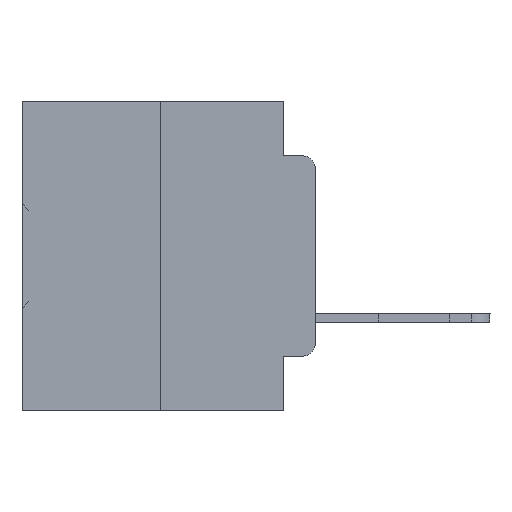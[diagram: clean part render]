
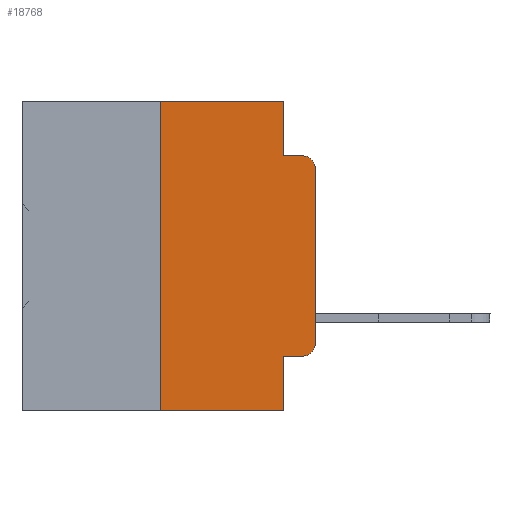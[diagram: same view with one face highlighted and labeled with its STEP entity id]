
A CAD part, left-side view. The second image highlights one B-rep face of the part: STEP entity #18768.
In plain terms, the highlighted planar face has unit normal (-1, 0, 0).
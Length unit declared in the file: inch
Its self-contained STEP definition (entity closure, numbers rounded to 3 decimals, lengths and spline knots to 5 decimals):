
#83 = EDGE_CURVE ( 'NONE', #33465, #11536, #35253, .T. ) ;
#577 = AXIS2_PLACEMENT_3D ( 'NONE', #12621, #35290, #26552 ) ;
#908 = CARTESIAN_POINT ( 'NONE',  ( 0., 0.473, 0. ) ) ;
#1136 = VERTEX_POINT ( 'NONE', #9105 ) ;
#1549 = LINE ( 'NONE', #27150, #31148 ) ;
#1655 = DIRECTION ( 'NONE',  ( 0., 0., -1. ) ) ;
#2420 = LINE ( 'NONE', #14021, #12284 ) ;
#2438 = ORIENTED_EDGE ( 'NONE', *, *, #31222, .T. ) ;
#2565 = DIRECTION ( 'NONE',  ( 0., 0., 1. ) ) ;
#2573 = LINE ( 'NONE', #4556, #23668 ) ;
#2904 = LINE ( 'NONE', #30087, #32514 ) ;
#3123 = AXIS2_PLACEMENT_3D ( 'NONE', #12083, #23395, #11851 ) ;
#3147 = VERTEX_POINT ( 'NONE', #8550 ) ;
#3445 = ORIENTED_EDGE ( 'NONE', *, *, #31385, .T. ) ;
#3495 = VERTEX_POINT ( 'NONE', #3893 ) ;
#3783 = DIRECTION ( 'NONE',  ( 1., 0., 0. ) ) ;
#3893 = CARTESIAN_POINT ( 'NONE',  ( 0., 0., -0.3915 ) ) ;
#4528 = ORIENTED_EDGE ( 'NONE', *, *, #83, .F. ) ;
#4556 = CARTESIAN_POINT ( 'NONE',  ( 0., 0.051, -0.0885 ) ) ;
#5218 = VECTOR ( 'NONE', #34963, 39.37008 ) ;
#6256 = VERTEX_POINT ( 'NONE', #10395 ) ;
#6557 = EDGE_CURVE ( 'NONE', #8669, #3147, #7519, .T. ) ;
#6685 = CARTESIAN_POINT ( 'NONE',  ( 0., 0.051, 0. ) ) ;
#7519 = LINE ( 'NONE', #17451, #8849 ) ;
#8210 = ORIENTED_EDGE ( 'NONE', *, *, #6557, .F. ) ;
#8270 = CARTESIAN_POINT ( 'NONE',  ( 0., 0.051, -0.0885 ) ) ;
#8550 = CARTESIAN_POINT ( 'NONE',  ( 0., 0.051, 0. ) ) ;
#8669 = VERTEX_POINT ( 'NONE', #10685 ) ;
#8849 = VECTOR ( 'NONE', #31893, 39.37008 ) ;
#9013 = LINE ( 'NONE', #33527, #32350 ) ;
#9105 = CARTESIAN_POINT ( 'NONE',  ( 0., 0., -0.1085 ) ) ;
#9427 = PLANE ( 'NONE',  #36697 ) ;
#10061 = EDGE_CURVE ( 'NONE', #1136, #10175, #16165, .T. ) ;
#10175 = VERTEX_POINT ( 'NONE', #18243 ) ;
#10395 = CARTESIAN_POINT ( 'NONE',  ( 0., 0.02, -0.4115 ) ) ;
#10685 = CARTESIAN_POINT ( 'NONE',  ( 0., 0.25, 0. ) ) ;
#11536 = VERTEX_POINT ( 'NONE', #26657 ) ;
#11851 = DIRECTION ( 'NONE',  ( 0., 0., -1. ) ) ;
#12083 = CARTESIAN_POINT ( 'NONE',  ( 0., 0.02, -0.1085 ) ) ;
#12284 = VECTOR ( 'NONE', #22689, 39.37008 ) ;
#12621 = CARTESIAN_POINT ( 'NONE',  ( 0., 0.02, -0.3915 ) ) ;
#12859 = DIRECTION ( 'NONE',  ( 0., 0., 1. ) ) ;
#14021 = CARTESIAN_POINT ( 'NONE',  ( 0., 0.051, -0.4115 ) ) ;
#14976 = CIRCLE ( 'NONE', #577, 0.02 ) ;
#15699 = DIRECTION ( 'NONE',  ( 0., -1., 0. ) ) ;
#16165 = CIRCLE ( 'NONE', #3123, 0.02 ) ;
#16654 = LINE ( 'NONE', #32131, #22017 ) ;
#17451 = CARTESIAN_POINT ( 'NONE',  ( 0., 0.473, 0. ) ) ;
#18243 = CARTESIAN_POINT ( 'NONE',  ( 0., 0.02, -0.0885 ) ) ;
#18655 = ORIENTED_EDGE ( 'NONE', *, *, #26228, .F. ) ;
#18768 = ADVANCED_FACE ( 'NONE', ( #36802 ), #9427, .F. ) ;
#18773 = CARTESIAN_POINT ( 'NONE',  ( 0., 0.051, -0.4115 ) ) ;
#22017 = VECTOR ( 'NONE', #1655, 39.37008 ) ;
#22689 = DIRECTION ( 'NONE',  ( 0., -1., 0. ) ) ;
#23395 = DIRECTION ( 'NONE',  ( -1., 0., 0. ) ) ;
#23668 = VECTOR ( 'NONE', #33487, 39.37008 ) ;
#23756 = ORIENTED_EDGE ( 'NONE', *, *, #36777, .T. ) ;
#23854 = DIRECTION ( 'NONE',  ( 0., 0., -1. ) ) ;
#24245 = ORIENTED_EDGE ( 'NONE', *, *, #10061, .T. ) ;
#24511 = VERTEX_POINT ( 'NONE', #33000 ) ;
#26228 = EDGE_CURVE ( 'NONE', #24511, #8669, #9013, .T. ) ;
#26552 = DIRECTION ( 'NONE',  ( 0., 0., -1. ) ) ;
#26657 = CARTESIAN_POINT ( 'NONE',  ( 0., 0.051, -0.5 ) ) ;
#27150 = CARTESIAN_POINT ( 'NONE',  ( 0., 0.473, -0.5 ) ) ;
#29152 = ORIENTED_EDGE ( 'NONE', *, *, #36086, .T. ) ;
#30087 = CARTESIAN_POINT ( 'NONE',  ( 0., 0., 0. ) ) ;
#30256 = ORIENTED_EDGE ( 'NONE', *, *, #32768, .F. ) ;
#31148 = VECTOR ( 'NONE', #15699, 39.37008 ) ;
#31222 = EDGE_CURVE ( 'NONE', #3495, #1136, #2904, .T. ) ;
#31385 = EDGE_CURVE ( 'NONE', #33465, #6256, #2420, .T. ) ;
#31648 = ORIENTED_EDGE ( 'NONE', *, *, #35061, .F. ) ;
#31893 = DIRECTION ( 'NONE',  ( 0., -1., 0. ) ) ;
#32131 = CARTESIAN_POINT ( 'NONE',  ( 0., 0.051, 0. ) ) ;
#32350 = VECTOR ( 'NONE', #2565, 39.37008 ) ;
#32514 = VECTOR ( 'NONE', #12859, 39.37008 ) ;
#32768 = EDGE_CURVE ( 'NONE', #3147, #35824, #16654, .T. ) ;
#33000 = CARTESIAN_POINT ( 'NONE',  ( 0., 0.25, -0.5 ) ) ;
#33465 = VERTEX_POINT ( 'NONE', #18773 ) ;
#33487 = DIRECTION ( 'NONE',  ( 0., -1., 0. ) ) ;
#33527 = CARTESIAN_POINT ( 'NONE',  ( 0., 0.25, 0. ) ) ;
#34963 = DIRECTION ( 'NONE',  ( 0., 0., -1. ) ) ;
#35061 = EDGE_CURVE ( 'NONE', #35824, #10175, #2573, .T. ) ;
#35253 = LINE ( 'NONE', #6685, #5218 ) ;
#35290 = DIRECTION ( 'NONE',  ( -1., 0., 0. ) ) ;
#35569 = EDGE_LOOP ( 'NONE', ( #2438, #24245, #31648, #30256, #8210, #18655, #23756, #4528, #3445, #29152 ) ) ;
#35824 = VERTEX_POINT ( 'NONE', #8270 ) ;
#36086 = EDGE_CURVE ( 'NONE', #6256, #3495, #14976, .T. ) ;
#36697 = AXIS2_PLACEMENT_3D ( 'NONE', #908, #3783, #23854 ) ;
#36777 = EDGE_CURVE ( 'NONE', #24511, #11536, #1549, .T. ) ;
#36802 = FACE_OUTER_BOUND ( 'NONE', #35569, .T. ) ;
